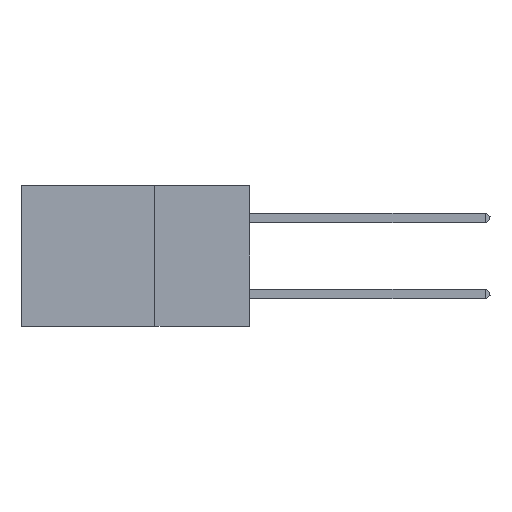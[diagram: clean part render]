
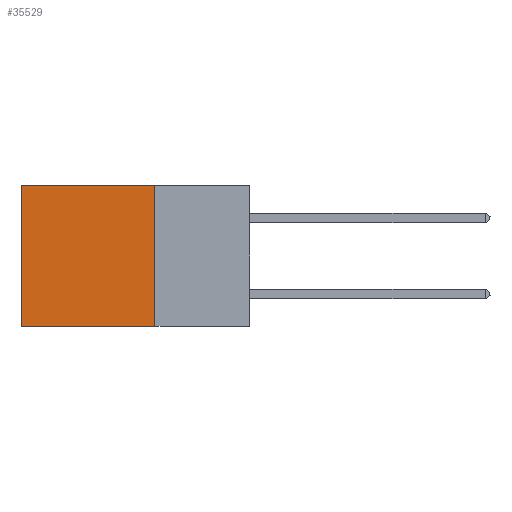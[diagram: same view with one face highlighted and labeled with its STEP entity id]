
A CAD part, left-side view. The second image highlights one B-rep face of the part: STEP entity #35529.
In plain terms, the highlighted planar face has unit normal (-1, 0, 0).
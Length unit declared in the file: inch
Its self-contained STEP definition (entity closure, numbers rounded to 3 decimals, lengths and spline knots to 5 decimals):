
#126 = DIRECTION ( 'NONE',  ( 0., 1., 0. ) ) ;
#314 = CARTESIAN_POINT ( 'NONE',  ( 0.2875, 0.6, 0. ) ) ;
#404 = VECTOR ( 'NONE', #11662, 39.37008 ) ;
#1137 = VERTEX_POINT ( 'NONE', #12109 ) ;
#1323 = LINE ( 'NONE', #29328, #404 ) ;
#2165 = CARTESIAN_POINT ( 'NONE',  ( 0.2875, 0.25, 0. ) ) ;
#2785 = ORIENTED_EDGE ( 'NONE', *, *, #18567, .T. ) ;
#3086 = CARTESIAN_POINT ( 'NONE',  ( 0.2875, 0.25, 0. ) ) ;
#3983 = LINE ( 'NONE', #26496, #22424 ) ;
#8323 = VERTEX_POINT ( 'NONE', #24726 ) ;
#10058 = VERTEX_POINT ( 'NONE', #3086 ) ;
#10428 = FACE_OUTER_BOUND ( 'NONE', #27370, .T. ) ;
#11662 = DIRECTION ( 'NONE',  ( 0., 1., 0. ) ) ;
#12109 = CARTESIAN_POINT ( 'NONE',  ( 0.2875, 0.6, -0.37 ) ) ;
#13571 = DIRECTION ( 'NONE',  ( 1., 0., 0. ) ) ;
#16478 = EDGE_CURVE ( 'NONE', #35315, #1137, #19269, .T. ) ;
#17266 = VECTOR ( 'NONE', #25659, 39.37008 ) ;
#18567 = EDGE_CURVE ( 'NONE', #10058, #35315, #3983, .T. ) ;
#18874 = CARTESIAN_POINT ( 'NONE',  ( 0.2875, 0.6, 0. ) ) ;
#19269 = LINE ( 'NONE', #314, #28051 ) ;
#19509 = DIRECTION ( 'NONE',  ( 0., 0., -1. ) ) ;
#21426 = LINE ( 'NONE', #34560, #17266 ) ;
#22424 = VECTOR ( 'NONE', #126, 39.37008 ) ;
#23603 = DIRECTION ( 'NONE',  ( 0., 0., -1. ) ) ;
#24726 = CARTESIAN_POINT ( 'NONE',  ( 0.2875, 0.25, -0.37 ) ) ;
#25659 = DIRECTION ( 'NONE',  ( 0., 0., -1. ) ) ;
#26496 = CARTESIAN_POINT ( 'NONE',  ( 0.2875, 0.25, 0. ) ) ;
#26597 = EDGE_CURVE ( 'NONE', #8323, #1137, #1323, .T. ) ;
#26891 = ORIENTED_EDGE ( 'NONE', *, *, #16478, .T. ) ;
#27370 = EDGE_LOOP ( 'NONE', ( #26891, #38144, #36468, #2785 ) ) ;
#28051 = VECTOR ( 'NONE', #23603, 39.37008 ) ;
#28287 = PLANE ( 'NONE',  #37405 ) ;
#29328 = CARTESIAN_POINT ( 'NONE',  ( 0.2875, 0.25, -0.37 ) ) ;
#30674 = EDGE_CURVE ( 'NONE', #10058, #8323, #21426, .T. ) ;
#34560 = CARTESIAN_POINT ( 'NONE',  ( 0.2875, 0.25, 0. ) ) ;
#35315 = VERTEX_POINT ( 'NONE', #18874 ) ;
#35529 = ADVANCED_FACE ( 'NONE', ( #10428 ), #28287, .F. ) ;
#36468 = ORIENTED_EDGE ( 'NONE', *, *, #30674, .F. ) ;
#37405 = AXIS2_PLACEMENT_3D ( 'NONE', #2165, #13571, #19509 ) ;
#38144 = ORIENTED_EDGE ( 'NONE', *, *, #26597, .F. ) ;
